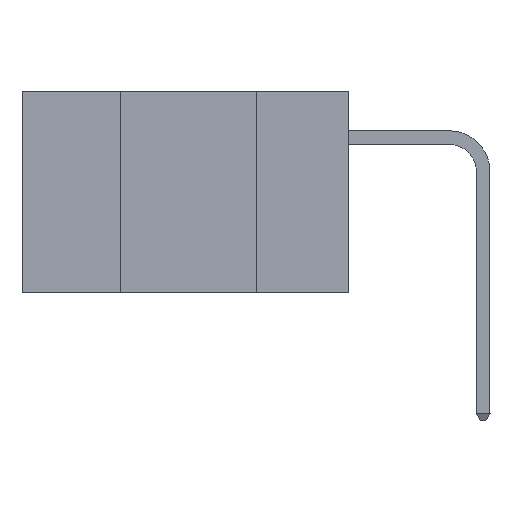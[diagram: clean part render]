
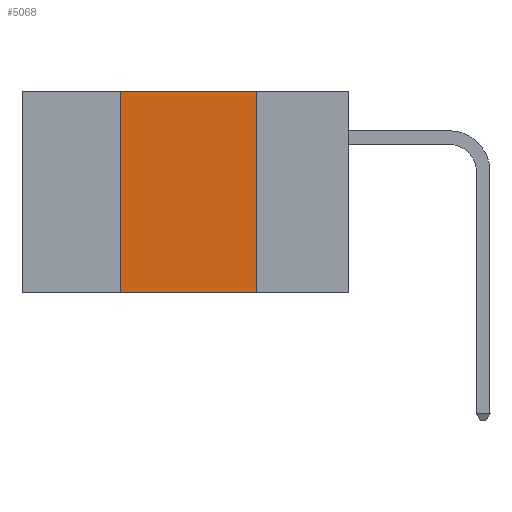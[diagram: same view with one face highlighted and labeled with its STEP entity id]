
A CAD part, left-side view. The second image highlights one B-rep face of the part: STEP entity #5068.
In plain terms, the highlighted planar face has unit normal (-1, 0, 0).
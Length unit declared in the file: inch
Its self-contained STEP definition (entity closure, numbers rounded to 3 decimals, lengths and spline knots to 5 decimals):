
#468 = DIRECTION ( 'NONE',  ( 1., 0., 0. ) ) ;
#2747 = CARTESIAN_POINT ( 'NONE',  ( 0., 0.17, -0.37 ) ) ;
#3212 = CARTESIAN_POINT ( 'NONE',  ( 0., 0.42, -0.37 ) ) ;
#3815 = VERTEX_POINT ( 'NONE', #3212 ) ;
#3818 = DIRECTION ( 'NONE',  ( 0., -1., 0. ) ) ;
#4167 = DIRECTION ( 'NONE',  ( 0., 0., -1. ) ) ;
#4654 = ORIENTED_EDGE ( 'NONE', *, *, #12896, .F. ) ;
#4901 = CARTESIAN_POINT ( 'NONE',  ( 0., 0.17, 0. ) ) ;
#5068 = ADVANCED_FACE ( 'NONE', ( #11108 ), #11343, .F. ) ;
#6306 = EDGE_CURVE ( 'NONE', #3815, #12577, #16698, .T. ) ;
#7628 = CARTESIAN_POINT ( 'NONE',  ( 0., 0.6, 0. ) ) ;
#7876 = CARTESIAN_POINT ( 'NONE',  ( 0., 0.6, -0.37 ) ) ;
#8441 = VECTOR ( 'NONE', #17876, 39.37008 ) ;
#9715 = VECTOR ( 'NONE', #3818, 39.37008 ) ;
#10845 = CARTESIAN_POINT ( 'NONE',  ( 0., 0.42, 0. ) ) ;
#11108 = FACE_OUTER_BOUND ( 'NONE', #17334, .T. ) ;
#11343 = PLANE ( 'NONE',  #18442 ) ;
#11477 = ORIENTED_EDGE ( 'NONE', *, *, #14023, .F. ) ;
#12577 = VERTEX_POINT ( 'NONE', #2747 ) ;
#12678 = CARTESIAN_POINT ( 'NONE',  ( 0., 0.17, 0. ) ) ;
#12896 = EDGE_CURVE ( 'NONE', #20613, #17528, #20291, .T. ) ;
#14023 = EDGE_CURVE ( 'NONE', #17528, #12577, #17676, .T. ) ;
#15620 = ORIENTED_EDGE ( 'NONE', *, *, #16095, .F. ) ;
#16095 = EDGE_CURVE ( 'NONE', #3815, #20613, #21477, .T. ) ;
#16698 = LINE ( 'NONE', #7876, #9715 ) ;
#17123 = VECTOR ( 'NONE', #17907, 39.37008 ) ;
#17334 = EDGE_LOOP ( 'NONE', ( #11477, #4654, #15620, #23351 ) ) ;
#17528 = VERTEX_POINT ( 'NONE', #12678 ) ;
#17676 = LINE ( 'NONE', #4901, #17123 ) ;
#17867 = VECTOR ( 'NONE', #18614, 39.37008 ) ;
#17876 = DIRECTION ( 'NONE',  ( 0., 0., 1. ) ) ;
#17907 = DIRECTION ( 'NONE',  ( 0., 0., -1. ) ) ;
#18442 = AXIS2_PLACEMENT_3D ( 'NONE', #20410, #468, #4167 ) ;
#18614 = DIRECTION ( 'NONE',  ( 0., -1., 0. ) ) ;
#20291 = LINE ( 'NONE', #7628, #17867 ) ;
#20410 = CARTESIAN_POINT ( 'NONE',  ( 0., 0.6, 0. ) ) ;
#20613 = VERTEX_POINT ( 'NONE', #22921 ) ;
#21477 = LINE ( 'NONE', #10845, #8441 ) ;
#22921 = CARTESIAN_POINT ( 'NONE',  ( 0., 0.42, 0. ) ) ;
#23351 = ORIENTED_EDGE ( 'NONE', *, *, #6306, .T. ) ;
